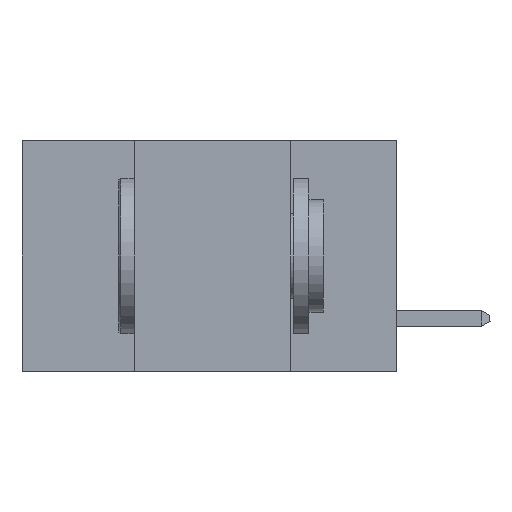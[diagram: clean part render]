
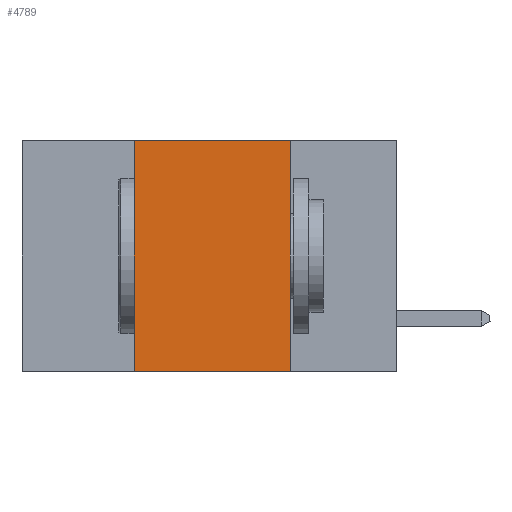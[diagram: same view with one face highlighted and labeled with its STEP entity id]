
A CAD part, left-side view. The second image highlights one B-rep face of the part: STEP entity #4789.
In plain terms, the highlighted planar face has unit normal (-1, 0, 0).
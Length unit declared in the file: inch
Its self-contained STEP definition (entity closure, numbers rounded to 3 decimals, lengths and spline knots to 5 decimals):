
#186 = VERTEX_POINT ( 'NONE', #13033 ) ;
#1064 = DIRECTION ( 'NONE',  ( 0., 0., 1. ) ) ;
#1133 = LINE ( 'NONE', #5183, #8396 ) ;
#3805 = CARTESIAN_POINT ( 'NONE',  ( 0., 0.42, 0. ) ) ;
#4789 = ADVANCED_FACE ( 'NONE', ( #22497 ), #17497, .F. ) ;
#4966 = AXIS2_PLACEMENT_3D ( 'NONE', #22131, #22263, #12376 ) ;
#5183 = CARTESIAN_POINT ( 'NONE',  ( 0., 0.42, 0. ) ) ;
#5487 = VERTEX_POINT ( 'NONE', #6384 ) ;
#5624 = ORIENTED_EDGE ( 'NONE', *, *, #25244, .F. ) ;
#5692 = ORIENTED_EDGE ( 'NONE', *, *, #19420, .F. ) ;
#6039 = ORIENTED_EDGE ( 'NONE', *, *, #17406, .F. ) ;
#6384 = CARTESIAN_POINT ( 'NONE',  ( 0., 0.42, -0.37 ) ) ;
#6618 = VERTEX_POINT ( 'NONE', #3805 ) ;
#6765 = ORIENTED_EDGE ( 'NONE', *, *, #13349, .T. ) ;
#7330 = CARTESIAN_POINT ( 'NONE',  ( 0., 0.6, 0. ) ) ;
#8306 = DIRECTION ( 'NONE',  ( 0., 0., -1. ) ) ;
#8346 = VECTOR ( 'NONE', #10196, 39.37008 ) ;
#8396 = VECTOR ( 'NONE', #1064, 39.37008 ) ;
#9984 = CARTESIAN_POINT ( 'NONE',  ( 0., 0.17, 0. ) ) ;
#10196 = DIRECTION ( 'NONE',  ( 0., -1., 0. ) ) ;
#10651 = VERTEX_POINT ( 'NONE', #9984 ) ;
#10967 = VECTOR ( 'NONE', #8306, 39.37008 ) ;
#11537 = VECTOR ( 'NONE', #19417, 39.37008 ) ;
#12282 = LINE ( 'NONE', #22272, #10967 ) ;
#12376 = DIRECTION ( 'NONE',  ( 0., 0., -1. ) ) ;
#13033 = CARTESIAN_POINT ( 'NONE',  ( 0., 0.17, -0.37 ) ) ;
#13349 = EDGE_CURVE ( 'NONE', #5487, #186, #13771, .T. ) ;
#13771 = LINE ( 'NONE', #20284, #8346 ) ;
#17406 = EDGE_CURVE ( 'NONE', #5487, #6618, #1133, .T. ) ;
#17497 = PLANE ( 'NONE',  #4966 ) ;
#18248 = EDGE_LOOP ( 'NONE', ( #5624, #5692, #6039, #6765 ) ) ;
#19417 = DIRECTION ( 'NONE',  ( 0., -1., 0. ) ) ;
#19420 = EDGE_CURVE ( 'NONE', #6618, #10651, #22821, .T. ) ;
#20284 = CARTESIAN_POINT ( 'NONE',  ( 0., 0.6, -0.37 ) ) ;
#22131 = CARTESIAN_POINT ( 'NONE',  ( 0., 0.6, 0. ) ) ;
#22263 = DIRECTION ( 'NONE',  ( 1., 0., 0. ) ) ;
#22272 = CARTESIAN_POINT ( 'NONE',  ( 0., 0.17, 0. ) ) ;
#22497 = FACE_OUTER_BOUND ( 'NONE', #18248, .T. ) ;
#22821 = LINE ( 'NONE', #7330, #11537 ) ;
#25244 = EDGE_CURVE ( 'NONE', #10651, #186, #12282, .T. ) ;
